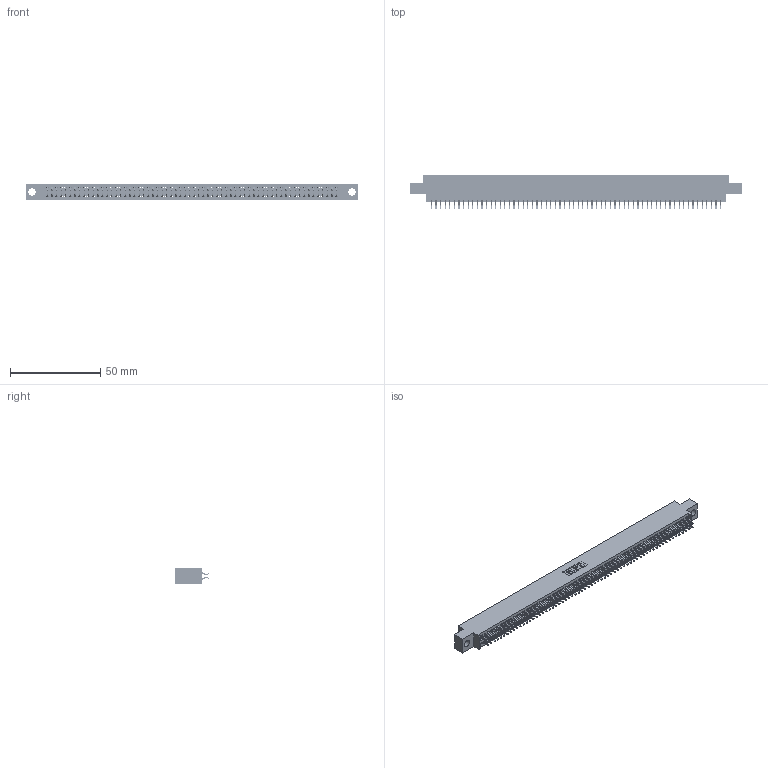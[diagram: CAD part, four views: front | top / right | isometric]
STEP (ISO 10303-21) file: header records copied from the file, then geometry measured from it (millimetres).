
FILE_DESCRIPTION (( 'STEP AP203' ), '1' );
FILE_NAME ('395-128-556-804.STEP', '2018-12-04T13:20:21', ( '' ), ( '' ), 'SwSTEP 2.0', 'SolidWorks 2016', '' );
FILE_SCHEMA (( 'CONFIG_CONTROL_DESIGN' ));
Length unit declared in the file: inch
Products named in the file (3): 395-128-556-804; 345 Part_0.170 Offset - 0.156 Dia-TH; 345-292-001_556 Tail
Assembly tree (129 placements, depth 2):
  395-128-556-804
    345 Part_0.170 Offset - 0.156 Dia-TH
    345-292-001_556 Tail  x128
Bounding box: 183.77 x 19.24 x 9.4 mm (x, y, z)
Volume: 17849.4 mm3; surface area: 26657.1 mm2
Topology: 129 solids, 129 shells, 7298 faces, 21729 edges, 14314 vertices
Faces by surface type: plane 4820, cylinder 2478
Entity records: 47609 total; most frequent: CARTESIAN_POINT 7976, ORIENTED_EDGE 7898, DIRECTION 6993, EDGE_CURVE 3949, VECTOR 3553, LINE 3553, VERTEX_POINT 2630, AXIS2_PLACEMENT_3D 1720
